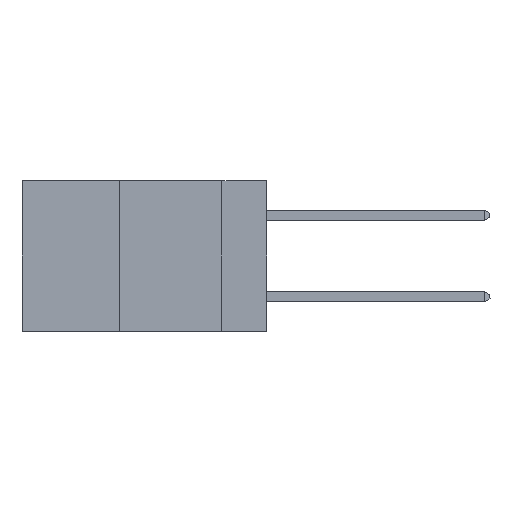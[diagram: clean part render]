
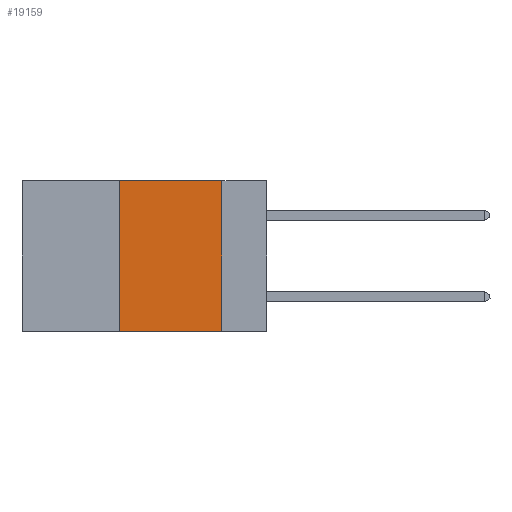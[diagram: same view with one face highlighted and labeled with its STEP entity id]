
A CAD part, left-side view. The second image highlights one B-rep face of the part: STEP entity #19159.
In plain terms, the highlighted planar face has unit normal (-1, 0, 0).
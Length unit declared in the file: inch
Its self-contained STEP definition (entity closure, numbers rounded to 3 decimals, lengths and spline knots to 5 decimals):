
#557 = ORIENTED_EDGE ( 'NONE', *, *, #2653, .F. ) ;
#736 = DIRECTION ( 'NONE',  ( 0., 0., -1. ) ) ;
#858 = VERTEX_POINT ( 'NONE', #2438 ) ;
#1043 = VERTEX_POINT ( 'NONE', #20992 ) ;
#1177 = ORIENTED_EDGE ( 'NONE', *, *, #3632, .F. ) ;
#1577 = CARTESIAN_POINT ( 'NONE',  ( 0., 0.36, -0.37 ) ) ;
#1691 = DIRECTION ( 'NONE',  ( 0., -1., 0. ) ) ;
#1942 = DIRECTION ( 'NONE',  ( 0., -1., 0. ) ) ;
#2393 = PLANE ( 'NONE',  #7400 ) ;
#2438 = CARTESIAN_POINT ( 'NONE',  ( 0., 0.11, -0.37 ) ) ;
#2653 = EDGE_CURVE ( 'NONE', #8475, #858, #3457, .T. ) ;
#3134 = ORIENTED_EDGE ( 'NONE', *, *, #6420, .F. ) ;
#3457 = LINE ( 'NONE', #11707, #22217 ) ;
#3560 = FACE_OUTER_BOUND ( 'NONE', #10343, .T. ) ;
#3632 = EDGE_CURVE ( 'NONE', #1043, #8475, #9255, .T. ) ;
#4036 = ORIENTED_EDGE ( 'NONE', *, *, #5232, .T. ) ;
#4358 = DIRECTION ( 'NONE',  ( 1., 0., 0. ) ) ;
#5134 = VECTOR ( 'NONE', #1942, 39.37008 ) ;
#5232 = EDGE_CURVE ( 'NONE', #21787, #858, #7016, .T. ) ;
#6392 = CARTESIAN_POINT ( 'NONE',  ( 0., 0.11, 0. ) ) ;
#6420 = EDGE_CURVE ( 'NONE', #21787, #1043, #6955, .T. ) ;
#6471 = VECTOR ( 'NONE', #1691, 39.37008 ) ;
#6955 = LINE ( 'NONE', #21060, #20391 ) ;
#7016 = LINE ( 'NONE', #22969, #6471 ) ;
#7400 = AXIS2_PLACEMENT_3D ( 'NONE', #13223, #4358, #16740 ) ;
#8475 = VERTEX_POINT ( 'NONE', #6392 ) ;
#9255 = LINE ( 'NONE', #12834, #5134 ) ;
#10343 = EDGE_LOOP ( 'NONE', ( #557, #1177, #3134, #4036 ) ) ;
#10624 = DIRECTION ( 'NONE',  ( 0., 0., 1. ) ) ;
#11707 = CARTESIAN_POINT ( 'NONE',  ( 0., 0.11, 0. ) ) ;
#12834 = CARTESIAN_POINT ( 'NONE',  ( 0., 0.6, 0. ) ) ;
#13223 = CARTESIAN_POINT ( 'NONE',  ( 0., 0.6, 0. ) ) ;
#16740 = DIRECTION ( 'NONE',  ( 0., 0., -1. ) ) ;
#19159 = ADVANCED_FACE ( 'NONE', ( #3560 ), #2393, .F. ) ;
#20391 = VECTOR ( 'NONE', #10624, 39.37008 ) ;
#20992 = CARTESIAN_POINT ( 'NONE',  ( 0., 0.36, 0. ) ) ;
#21060 = CARTESIAN_POINT ( 'NONE',  ( 0., 0.36, 0. ) ) ;
#21787 = VERTEX_POINT ( 'NONE', #1577 ) ;
#22217 = VECTOR ( 'NONE', #736, 39.37008 ) ;
#22969 = CARTESIAN_POINT ( 'NONE',  ( 0., 0.6, -0.37 ) ) ;
